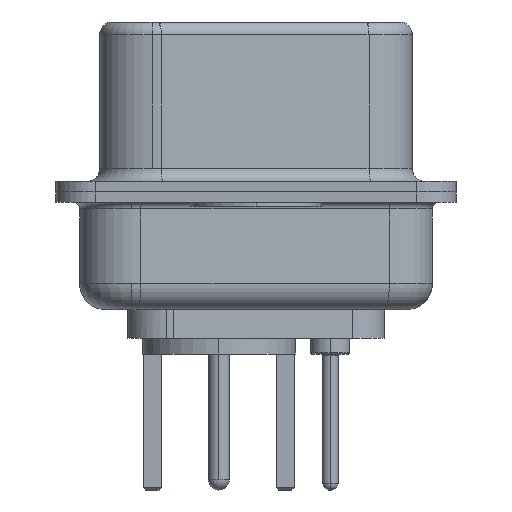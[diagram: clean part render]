
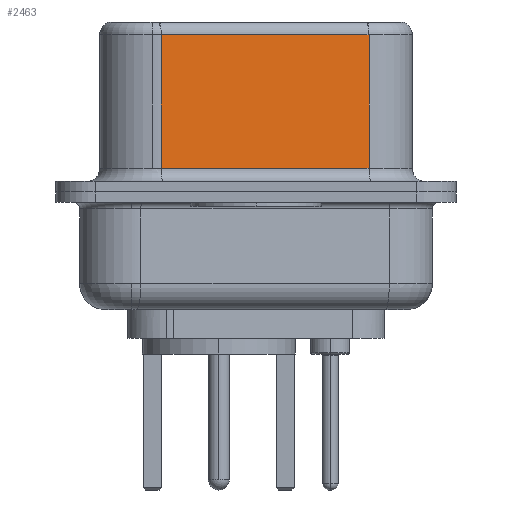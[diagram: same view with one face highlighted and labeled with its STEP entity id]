
A CAD part, left-side view. The second image highlights one B-rep face of the part: STEP entity #2463.
In plain terms, the highlighted planar face has unit normal (-0.985, -0.174, 0).
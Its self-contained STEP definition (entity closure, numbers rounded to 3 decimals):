
#696 = AXIS2_PLACEMENT_3D ( 'NONE', #17068, #19383, #9286 ) ;
#1550 = LINE ( 'NONE', #18937, #14592 ) ;
#2053 = ORIENTED_EDGE ( 'NONE', *, *, #10570, .F. ) ;
#2095 = CARTESIAN_POINT ( 'NONE',  ( 5.132, -4.322, 0.9 ) ) ;
#2284 = EDGE_CURVE ( 'NONE', #11428, #18864, #1550, .T. ) ;
#2463 = ADVANCED_FACE ( 'NONE', ( #7471 ), #14118, .F. ) ;
#2921 = CARTESIAN_POINT ( 'NONE',  ( 5.132, -4.322, 6.52 ) ) ;
#3416 = EDGE_CURVE ( 'NONE', #10607, #11303, #12961, .T. ) ;
#4940 = LINE ( 'NONE', #7625, #9464 ) ;
#6424 = DIRECTION ( 'NONE',  ( 0., 0., -1. ) ) ;
#7413 = ORIENTED_EDGE ( 'NONE', *, *, #3416, .T. ) ;
#7471 = FACE_OUTER_BOUND ( 'NONE', #14837, .T. ) ;
#7553 = DIRECTION ( 'NONE',  ( -0.174, 0.985, 0. ) ) ;
#7625 = CARTESIAN_POINT ( 'NONE',  ( 3.73, 3.628, 6.52 ) ) ;
#8501 = VECTOR ( 'NONE', #7553, 1000. ) ;
#9286 = DIRECTION ( 'NONE',  ( -0.174, 0.985, 0. ) ) ;
#9464 = VECTOR ( 'NONE', #19382, 1000. ) ;
#10385 = EDGE_CURVE ( 'NONE', #11303, #11428, #4940, .T. ) ;
#10570 = EDGE_CURVE ( 'NONE', #10607, #18864, #18692, .T. ) ;
#10607 = VERTEX_POINT ( 'NONE', #14909 ) ;
#11303 = VERTEX_POINT ( 'NONE', #20077 ) ;
#11428 = VERTEX_POINT ( 'NONE', #13748 ) ;
#11913 = CARTESIAN_POINT ( 'NONE',  ( 5.132, -4.322, 6.02 ) ) ;
#12961 = LINE ( 'NONE', #11913, #8501 ) ;
#13748 = CARTESIAN_POINT ( 'NONE',  ( 3.73, 3.628, 0.9 ) ) ;
#14118 = PLANE ( 'NONE',  #696 ) ;
#14197 = VECTOR ( 'NONE', #6424, 1000. ) ;
#14592 = VECTOR ( 'NONE', #21090, 1000. ) ;
#14837 = EDGE_LOOP ( 'NONE', ( #2053, #7413, #16813, #19876 ) ) ;
#14909 = CARTESIAN_POINT ( 'NONE',  ( 5.132, -4.322, 6.02 ) ) ;
#16813 = ORIENTED_EDGE ( 'NONE', *, *, #10385, .T. ) ;
#17068 = CARTESIAN_POINT ( 'NONE',  ( 5.132, -4.322, 6.52 ) ) ;
#18692 = LINE ( 'NONE', #2921, #14197 ) ;
#18864 = VERTEX_POINT ( 'NONE', #2095 ) ;
#18937 = CARTESIAN_POINT ( 'NONE',  ( 5.132, -4.322, 0.9 ) ) ;
#19382 = DIRECTION ( 'NONE',  ( 0., 0., -1. ) ) ;
#19383 = DIRECTION ( 'NONE',  ( 0.985, 0.174, 0. ) ) ;
#19876 = ORIENTED_EDGE ( 'NONE', *, *, #2284, .T. ) ;
#20077 = CARTESIAN_POINT ( 'NONE',  ( 3.73, 3.628, 6.02 ) ) ;
#21090 = DIRECTION ( 'NONE',  ( 0.174, -0.985, 0. ) ) ;
